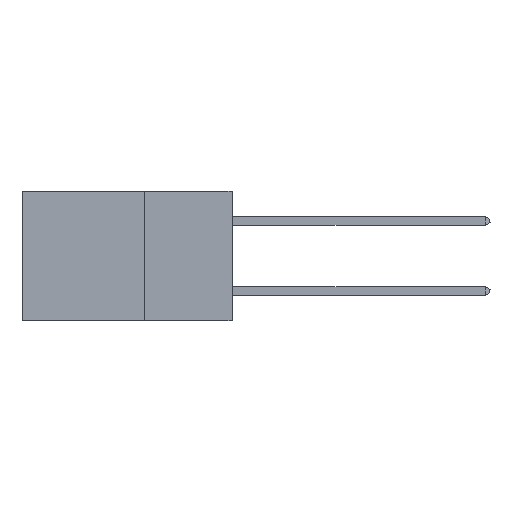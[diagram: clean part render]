
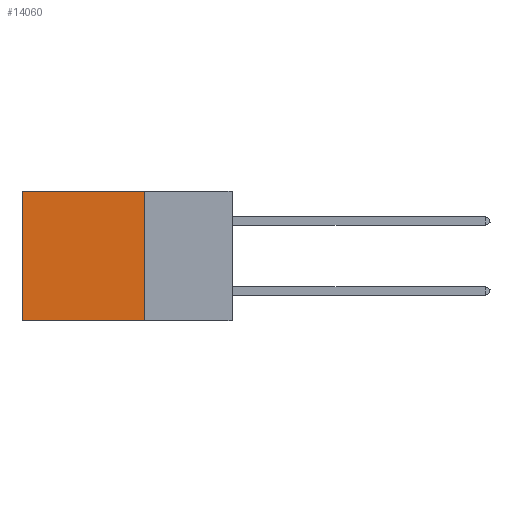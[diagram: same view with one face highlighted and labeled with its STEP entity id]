
A CAD part, left-side view. The second image highlights one B-rep face of the part: STEP entity #14060.
In plain terms, the highlighted planar face has unit normal (-1, 0, 0).
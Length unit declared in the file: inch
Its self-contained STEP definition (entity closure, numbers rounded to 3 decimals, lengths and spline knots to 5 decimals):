
#193 = CARTESIAN_POINT ( 'NONE',  ( 0.2875, 0.25, 0. ) ) ;
#301 = AXIS2_PLACEMENT_3D ( 'NONE', #193, #3171, #12896 ) ;
#1065 = VECTOR ( 'NONE', #9739, 39.37008 ) ;
#1679 = PLANE ( 'NONE',  #301 ) ;
#1897 = DIRECTION ( 'NONE',  ( 0., 1., 0. ) ) ;
#2312 = DIRECTION ( 'NONE',  ( 0., 0., -1. ) ) ;
#2345 = EDGE_CURVE ( 'NONE', #8442, #8381, #9100, .T. ) ;
#3171 = DIRECTION ( 'NONE',  ( 1., 0., 0. ) ) ;
#3902 = VECTOR ( 'NONE', #5764, 39.37008 ) ;
#4680 = CARTESIAN_POINT ( 'NONE',  ( 0.2875, 0.6, 0. ) ) ;
#5002 = LINE ( 'NONE', #11531, #1065 ) ;
#5404 = EDGE_CURVE ( 'NONE', #5542, #7737, #5002, .T. ) ;
#5542 = VERTEX_POINT ( 'NONE', #7799 ) ;
#5764 = DIRECTION ( 'NONE',  ( 0., 1., 0. ) ) ;
#6889 = ORIENTED_EDGE ( 'NONE', *, *, #2345, .T. ) ;
#7093 = ORIENTED_EDGE ( 'NONE', *, *, #13922, .F. ) ;
#7497 = ORIENTED_EDGE ( 'NONE', *, *, #5404, .F. ) ;
#7737 = VERTEX_POINT ( 'NONE', #8181 ) ;
#7738 = LINE ( 'NONE', #14438, #10536 ) ;
#7799 = CARTESIAN_POINT ( 'NONE',  ( 0.2875, 0.25, 0. ) ) ;
#7949 = ORIENTED_EDGE ( 'NONE', *, *, #9409, .T. ) ;
#8181 = CARTESIAN_POINT ( 'NONE',  ( 0.2875, 0.25, -0.37 ) ) ;
#8381 = VERTEX_POINT ( 'NONE', #16370 ) ;
#8442 = VERTEX_POINT ( 'NONE', #9895 ) ;
#9100 = LINE ( 'NONE', #4680, #9529 ) ;
#9199 = FACE_OUTER_BOUND ( 'NONE', #15676, .T. ) ;
#9409 = EDGE_CURVE ( 'NONE', #5542, #8442, #7738, .T. ) ;
#9529 = VECTOR ( 'NONE', #2312, 39.37008 ) ;
#9739 = DIRECTION ( 'NONE',  ( 0., 0., -1. ) ) ;
#9895 = CARTESIAN_POINT ( 'NONE',  ( 0.2875, 0.6, 0. ) ) ;
#10536 = VECTOR ( 'NONE', #1897, 39.37008 ) ;
#11531 = CARTESIAN_POINT ( 'NONE',  ( 0.2875, 0.25, 0. ) ) ;
#12896 = DIRECTION ( 'NONE',  ( 0., 0., -1. ) ) ;
#13922 = EDGE_CURVE ( 'NONE', #7737, #8381, #14852, .T. ) ;
#14060 = ADVANCED_FACE ( 'NONE', ( #9199 ), #1679, .F. ) ;
#14438 = CARTESIAN_POINT ( 'NONE',  ( 0.2875, 0.25, 0. ) ) ;
#14852 = LINE ( 'NONE', #17715, #3902 ) ;
#15676 = EDGE_LOOP ( 'NONE', ( #6889, #7093, #7497, #7949 ) ) ;
#16370 = CARTESIAN_POINT ( 'NONE',  ( 0.2875, 0.6, -0.37 ) ) ;
#17715 = CARTESIAN_POINT ( 'NONE',  ( 0.2875, 0.25, -0.37 ) ) ;
